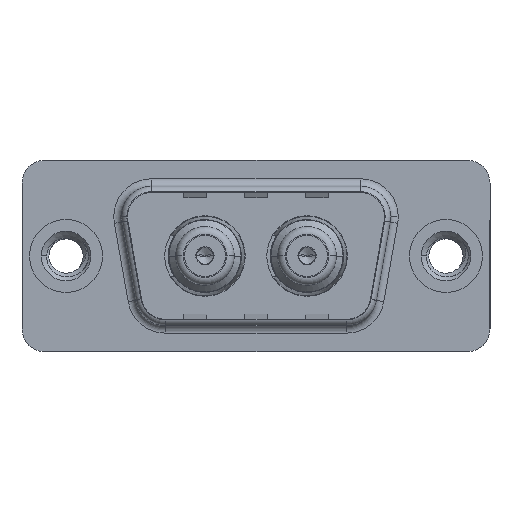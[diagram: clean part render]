
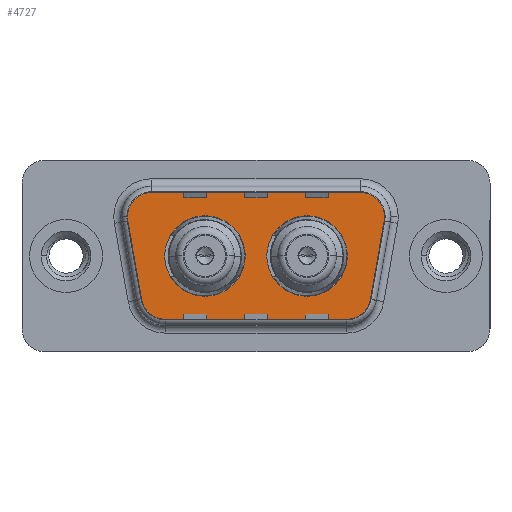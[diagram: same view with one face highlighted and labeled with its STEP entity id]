
A CAD part, top view. The second image highlights one B-rep face of the part: STEP entity #4727.
In plain terms, the highlighted planar face has unit normal (0, 0, 1).
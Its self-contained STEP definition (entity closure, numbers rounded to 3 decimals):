
#47 = CARTESIAN_POINT ( 'NONE',  ( 5.436, 4.9, 0. ) ) ;
#223 = FACE_BOUND ( 'NONE', #2903, .T. ) ;
#249 = CIRCLE ( 'NONE', #11459, 2.65 ) ;
#372 = EDGE_CURVE ( 'NONE', #4337, #2599, #6830, .T. ) ;
#383 = ORIENTED_EDGE ( 'NONE', *, *, #6204, .F. ) ;
#399 = VERTEX_POINT ( 'NONE', #12287 ) ;
#649 = VECTOR ( 'NONE', #13219, 1000. ) ;
#1127 = CIRCLE ( 'NONE', #10827, 2. ) ;
#1306 = CIRCLE ( 'NONE', #13756, 2. ) ;
#1662 = CIRCLE ( 'NONE', #7786, 2. ) ;
#1780 = EDGE_CURVE ( 'NONE', #4687, #4353, #9397, .T. ) ;
#1798 = EDGE_CURVE ( 'NONE', #4846, #399, #9735, .T. ) ;
#2191 = LINE ( 'NONE', #13985, #13765 ) ;
#2273 = CARTESIAN_POINT ( 'NONE',  ( 20.511, -3.247, 0. ) ) ;
#2323 = EDGE_CURVE ( 'NONE', #399, #11666, #1662, .T. ) ;
#2599 = VERTEX_POINT ( 'NONE', #2675 ) ;
#2675 = CARTESIAN_POINT ( 'NONE',  ( 3.466, 2.553, 0. ) ) ;
#2903 = EDGE_LOOP ( 'NONE', ( #12499, #5691 ) ) ;
#2982 = EDGE_CURVE ( 'NONE', #11666, #12646, #1306, .T. ) ;
#3085 = CARTESIAN_POINT ( 'NONE',  ( 19.564, 2.9, 0. ) ) ;
#3120 = DIRECTION ( 'NONE',  ( 0., 0., 1. ) ) ;
#3153 = VERTEX_POINT ( 'NONE', #13245 ) ;
#3177 = CARTESIAN_POINT ( 'NONE',  ( 6.459, -2.9, 0. ) ) ;
#3335 = EDGE_CURVE ( 'NONE', #3153, #4846, #5920, .T. ) ;
#3345 = DIRECTION ( 'NONE',  ( -1., 0., 0. ) ) ;
#3346 = CARTESIAN_POINT ( 'NONE',  ( 4.489, -3.247, 0. ) ) ;
#3424 = ORIENTED_EDGE ( 'NONE', *, *, #9503, .T. ) ;
#3497 = FACE_BOUND ( 'NONE', #9975, .T. ) ;
#3595 = AXIS2_PLACEMENT_3D ( 'NONE', #12768, #6262, #13857 ) ;
#3825 = ORIENTED_EDGE ( 'NONE', *, *, #9172, .T. ) ;
#3949 = VECTOR ( 'NONE', #3345, 1000. ) ;
#4023 = DIRECTION ( 'NONE',  ( 1., 0., 0. ) ) ;
#4039 = DIRECTION ( 'NONE',  ( 0., 0., 1. ) ) ;
#4187 = CARTESIAN_POINT ( 'NONE',  ( 18.541, -2.9, 0. ) ) ;
#4280 = PLANE ( 'NONE',  #6784 ) ;
#4302 = DIRECTION ( 'NONE',  ( -1., 0., 0. ) ) ;
#4337 = VERTEX_POINT ( 'NONE', #8764 ) ;
#4353 = VERTEX_POINT ( 'NONE', #8718 ) ;
#4601 = CARTESIAN_POINT ( 'NONE',  ( 11.79, 0., 0. ) ) ;
#4687 = VERTEX_POINT ( 'NONE', #4601 ) ;
#4727 = ADVANCED_FACE ( 'NONE', ( #3497, #223, #6035 ), #4280, .T. ) ;
#4846 = VERTEX_POINT ( 'NONE', #2273 ) ;
#4873 = CARTESIAN_POINT ( 'NONE',  ( 18.51, 0., 0. ) ) ;
#5240 = AXIS2_PLACEMENT_3D ( 'NONE', #10576, #10559, #10535 ) ;
#5403 = AXIS2_PLACEMENT_3D ( 'NONE', #13181, #13161, #13118 ) ;
#5691 = ORIENTED_EDGE ( 'NONE', *, *, #11376, .F. ) ;
#5717 = VERTEX_POINT ( 'NONE', #9651 ) ;
#5739 = CARTESIAN_POINT ( 'NONE',  ( 9.14, 0., 0. ) ) ;
#5871 = DIRECTION ( 'NONE',  ( -1., 0., 0. ) ) ;
#5913 = DIRECTION ( 'NONE',  ( 0., 0., 1. ) ) ;
#5920 = CIRCLE ( 'NONE', #5240, 2. ) ;
#5926 = CARTESIAN_POINT ( 'NONE',  ( 19.564, 2.9, 0. ) ) ;
#6035 = FACE_OUTER_BOUND ( 'NONE', #10310, .T. ) ;
#6176 = CIRCLE ( 'NONE', #12681, 2.65 ) ;
#6204 = EDGE_CURVE ( 'NONE', #5717, #6402, #6176, .T. ) ;
#6262 = DIRECTION ( 'NONE',  ( 0., 0., 1. ) ) ;
#6402 = VERTEX_POINT ( 'NONE', #4873 ) ;
#6525 = CARTESIAN_POINT ( 'NONE',  ( 6.459, -4.9, 0. ) ) ;
#6620 = ORIENTED_EDGE ( 'NONE', *, *, #372, .T. ) ;
#6677 = CIRCLE ( 'NONE', #3595, 2.65 ) ;
#6751 = AXIS2_PLACEMENT_3D ( 'NONE', #12590, #12561, #12518 ) ;
#6754 = ORIENTED_EDGE ( 'NONE', *, *, #3335, .T. ) ;
#6784 = AXIS2_PLACEMENT_3D ( 'NONE', #4187, #4039, #4023 ) ;
#6830 = CIRCLE ( 'NONE', #6751, 2. ) ;
#6835 = DIRECTION ( 'NONE',  ( 1., 0., 0. ) ) ;
#6838 = DIRECTION ( 'NONE',  ( 1., 0., 0. ) ) ;
#7010 = EDGE_CURVE ( 'NONE', #6402, #5717, #6677, .T. ) ;
#7285 = EDGE_CURVE ( 'NONE', #12646, #4337, #9758, .T. ) ;
#7521 = DIRECTION ( 'NONE',  ( 0.174, -0.985, 0. ) ) ;
#7786 = AXIS2_PLACEMENT_3D ( 'NONE', #5926, #5913, #5871 ) ;
#7936 = CARTESIAN_POINT ( 'NONE',  ( 6.459, -4.9, 0. ) ) ;
#7996 = ORIENTED_EDGE ( 'NONE', *, *, #2323, .T. ) ;
#8070 = ORIENTED_EDGE ( 'NONE', *, *, #7010, .F. ) ;
#8181 = LINE ( 'NONE', #7936, #10389 ) ;
#8718 = CARTESIAN_POINT ( 'NONE',  ( 6.49, 0., 0. ) ) ;
#8764 = CARTESIAN_POINT ( 'NONE',  ( 5.436, 4.9, 0. ) ) ;
#8858 = ORIENTED_EDGE ( 'NONE', *, *, #1798, .T. ) ;
#9172 = EDGE_CURVE ( 'NONE', #2599, #9325, #2191, .T. ) ;
#9217 = ORIENTED_EDGE ( 'NONE', *, *, #10494, .T. ) ;
#9325 = VERTEX_POINT ( 'NONE', #3346 ) ;
#9393 = DIRECTION ( 'NONE',  ( 1., 0., 0. ) ) ;
#9397 = CIRCLE ( 'NONE', #5403, 2.65 ) ;
#9503 = EDGE_CURVE ( 'NONE', #9957, #3153, #8181, .T. ) ;
#9518 = DIRECTION ( 'NONE',  ( 0., 0., 1. ) ) ;
#9561 = CARTESIAN_POINT ( 'NONE',  ( 15.86, 0., 0. ) ) ;
#9651 = CARTESIAN_POINT ( 'NONE',  ( 13.21, 0., 0. ) ) ;
#9735 = LINE ( 'NONE', #13268, #649 ) ;
#9758 = LINE ( 'NONE', #47, #3949 ) ;
#9957 = VERTEX_POINT ( 'NONE', #6525 ) ;
#9975 = EDGE_LOOP ( 'NONE', ( #8070, #383 ) ) ;
#10310 = EDGE_LOOP ( 'NONE', ( #6754, #8858, #7996, #12296, #12149, #6620, #3825, #9217, #3424 ) ) ;
#10389 = VECTOR ( 'NONE', #6835, 1000. ) ;
#10450 = CARTESIAN_POINT ( 'NONE',  ( 19.564, 4.9, 0. ) ) ;
#10494 = EDGE_CURVE ( 'NONE', #9325, #9957, #1127, .T. ) ;
#10535 = DIRECTION ( 'NONE',  ( 1., 0., 0. ) ) ;
#10559 = DIRECTION ( 'NONE',  ( 0., 0., 1. ) ) ;
#10576 = CARTESIAN_POINT ( 'NONE',  ( 18.541, -2.9, 0. ) ) ;
#10806 = DIRECTION ( 'NONE',  ( 0., 0., 1. ) ) ;
#10827 = AXIS2_PLACEMENT_3D ( 'NONE', #3177, #10806, #4302 ) ;
#11376 = EDGE_CURVE ( 'NONE', #4353, #4687, #249, .T. ) ;
#11459 = AXIS2_PLACEMENT_3D ( 'NONE', #5739, #13314, #6838 ) ;
#11504 = DIRECTION ( 'NONE',  ( -1., 0., 0. ) ) ;
#11666 = VERTEX_POINT ( 'NONE', #12610 ) ;
#12149 = ORIENTED_EDGE ( 'NONE', *, *, #7285, .T. ) ;
#12287 = CARTESIAN_POINT ( 'NONE',  ( 21.534, 2.553, 0. ) ) ;
#12296 = ORIENTED_EDGE ( 'NONE', *, *, #2982, .T. ) ;
#12499 = ORIENTED_EDGE ( 'NONE', *, *, #1780, .F. ) ;
#12518 = DIRECTION ( 'NONE',  ( 1., 0., 0. ) ) ;
#12561 = DIRECTION ( 'NONE',  ( 0., 0., 1. ) ) ;
#12590 = CARTESIAN_POINT ( 'NONE',  ( 5.436, 2.9, 0. ) ) ;
#12610 = CARTESIAN_POINT ( 'NONE',  ( 21.564, 2.9, 0. ) ) ;
#12646 = VERTEX_POINT ( 'NONE', #10450 ) ;
#12681 = AXIS2_PLACEMENT_3D ( 'NONE', #9561, #9518, #9393 ) ;
#12768 = CARTESIAN_POINT ( 'NONE',  ( 15.86, 0., 0. ) ) ;
#13118 = DIRECTION ( 'NONE',  ( 1., 0., 0. ) ) ;
#13161 = DIRECTION ( 'NONE',  ( 0., 0., 1. ) ) ;
#13181 = CARTESIAN_POINT ( 'NONE',  ( 9.14, 0., 0. ) ) ;
#13219 = DIRECTION ( 'NONE',  ( 0.174, 0.985, 0. ) ) ;
#13245 = CARTESIAN_POINT ( 'NONE',  ( 18.541, -4.9, 0. ) ) ;
#13268 = CARTESIAN_POINT ( 'NONE',  ( 21.534, 2.553, 0. ) ) ;
#13314 = DIRECTION ( 'NONE',  ( 0., 0., 1. ) ) ;
#13756 = AXIS2_PLACEMENT_3D ( 'NONE', #3085, #3120, #11504 ) ;
#13765 = VECTOR ( 'NONE', #7521, 1000. ) ;
#13857 = DIRECTION ( 'NONE',  ( 1., 0., 0. ) ) ;
#13985 = CARTESIAN_POINT ( 'NONE',  ( 3.466, 2.553, 0. ) ) ;
